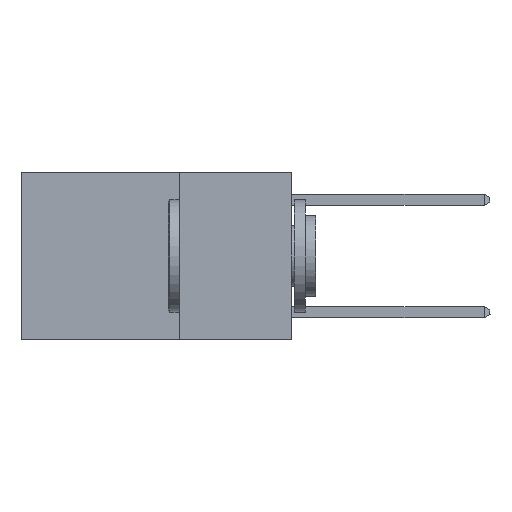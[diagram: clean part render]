
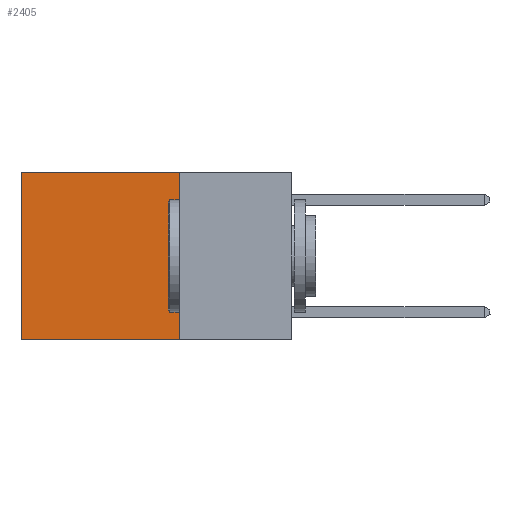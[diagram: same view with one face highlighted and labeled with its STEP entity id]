
A CAD part, left-side view. The second image highlights one B-rep face of the part: STEP entity #2405.
In plain terms, the highlighted planar face has unit normal (-1, 0, 0).
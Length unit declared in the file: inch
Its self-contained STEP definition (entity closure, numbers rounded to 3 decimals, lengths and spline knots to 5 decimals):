
#455 = VERTEX_POINT ( 'NONE', #2676 ) ;
#837 = VERTEX_POINT ( 'NONE', #23373 ) ;
#948 = ORIENTED_EDGE ( 'NONE', *, *, #23958, .F. ) ;
#1244 = EDGE_LOOP ( 'NONE', ( #11778, #948, #24700, #21342 ) ) ;
#1872 = LINE ( 'NONE', #12408, #5476 ) ;
#2405 = ADVANCED_FACE ( 'NONE', ( #4288 ), #19183, .F. ) ;
#2676 = CARTESIAN_POINT ( 'NONE',  ( 0.2625, 0.25, -0.37 ) ) ;
#4288 = FACE_OUTER_BOUND ( 'NONE', #1244, .T. ) ;
#4354 = LINE ( 'NONE', #12692, #20300 ) ;
#4543 = VERTEX_POINT ( 'NONE', #7797 ) ;
#5476 = VECTOR ( 'NONE', #23312, 39.37008 ) ;
#7797 = CARTESIAN_POINT ( 'NONE',  ( 0.2625, 0.25, 0. ) ) ;
#9295 = DIRECTION ( 'NONE',  ( 0., 0., -1. ) ) ;
#10498 = DIRECTION ( 'NONE',  ( 0., 0., -1. ) ) ;
#10679 = AXIS2_PLACEMENT_3D ( 'NONE', #23000, #20950, #21087 ) ;
#11741 = LINE ( 'NONE', #20057, #21366 ) ;
#11778 = ORIENTED_EDGE ( 'NONE', *, *, #15866, .T. ) ;
#12408 = CARTESIAN_POINT ( 'NONE',  ( 0.2625, 0.25, 0. ) ) ;
#12692 = CARTESIAN_POINT ( 'NONE',  ( 0.2625, 0.25, 0. ) ) ;
#12902 = LINE ( 'NONE', #23262, #13306 ) ;
#13306 = VECTOR ( 'NONE', #21082, 39.37008 ) ;
#15866 = EDGE_CURVE ( 'NONE', #837, #26927, #11741, .T. ) ;
#19183 = PLANE ( 'NONE',  #10679 ) ;
#20057 = CARTESIAN_POINT ( 'NONE',  ( 0.2625, 0.6, 0. ) ) ;
#20300 = VECTOR ( 'NONE', #10498, 39.37008 ) ;
#20950 = DIRECTION ( 'NONE',  ( 1., 0., 0. ) ) ;
#21082 = DIRECTION ( 'NONE',  ( 0., 1., 0. ) ) ;
#21087 = DIRECTION ( 'NONE',  ( 0., 0., -1. ) ) ;
#21342 = ORIENTED_EDGE ( 'NONE', *, *, #26678, .T. ) ;
#21366 = VECTOR ( 'NONE', #9295, 39.37008 ) ;
#22472 = CARTESIAN_POINT ( 'NONE',  ( 0.2625, 0.6, -0.37 ) ) ;
#23000 = CARTESIAN_POINT ( 'NONE',  ( 0.2625, 0.25, 0. ) ) ;
#23262 = CARTESIAN_POINT ( 'NONE',  ( 0.2625, 0.25, -0.37 ) ) ;
#23312 = DIRECTION ( 'NONE',  ( 0., 1., 0. ) ) ;
#23373 = CARTESIAN_POINT ( 'NONE',  ( 0.2625, 0.6, 0. ) ) ;
#23958 = EDGE_CURVE ( 'NONE', #455, #26927, #12902, .T. ) ;
#24700 = ORIENTED_EDGE ( 'NONE', *, *, #24849, .F. ) ;
#24849 = EDGE_CURVE ( 'NONE', #4543, #455, #4354, .T. ) ;
#26678 = EDGE_CURVE ( 'NONE', #4543, #837, #1872, .T. ) ;
#26927 = VERTEX_POINT ( 'NONE', #22472 ) ;
